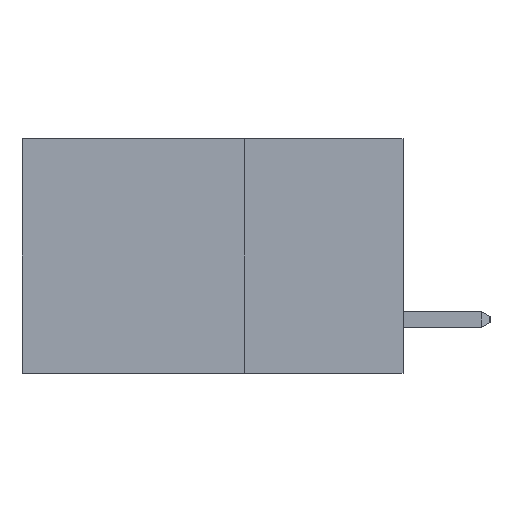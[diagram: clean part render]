
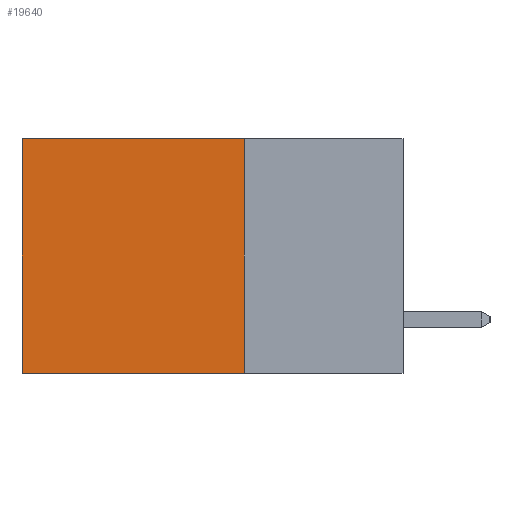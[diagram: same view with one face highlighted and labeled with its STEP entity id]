
A CAD part, left-side view. The second image highlights one B-rep face of the part: STEP entity #19640.
In plain terms, the highlighted planar face has unit normal (-1, 0, 0).
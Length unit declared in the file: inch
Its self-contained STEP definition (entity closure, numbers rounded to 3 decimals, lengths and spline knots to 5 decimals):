
#230 = EDGE_CURVE ( 'NONE', #2887, #5581, #7530, .T. ) ;
#419 = DIRECTION ( 'NONE',  ( 0., 1., 0. ) ) ;
#2053 = LINE ( 'NONE', #7343, #9746 ) ;
#2847 = LINE ( 'NONE', #5994, #10542 ) ;
#2887 = VERTEX_POINT ( 'NONE', #11896 ) ;
#3001 = ORIENTED_EDGE ( 'NONE', *, *, #4928, .F. ) ;
#3057 = VECTOR ( 'NONE', #419, 39.37008 ) ;
#4457 = CARTESIAN_POINT ( 'NONE',  ( 0.2875, 0.25, 0. ) ) ;
#4928 = EDGE_CURVE ( 'NONE', #5581, #10847, #2053, .T. ) ;
#5384 = ORIENTED_EDGE ( 'NONE', *, *, #10933, .T. ) ;
#5581 = VERTEX_POINT ( 'NONE', #11566 ) ;
#5994 = CARTESIAN_POINT ( 'NONE',  ( 0.2875, 0.6, 0. ) ) ;
#6035 = DIRECTION ( 'NONE',  ( 1., 0., 0. ) ) ;
#7012 = LINE ( 'NONE', #19492, #3057 ) ;
#7343 = CARTESIAN_POINT ( 'NONE',  ( 0.2875, 0.25, -0.37 ) ) ;
#7530 = LINE ( 'NONE', #17362, #8011 ) ;
#8011 = VECTOR ( 'NONE', #12726, 39.37008 ) ;
#8301 = CARTESIAN_POINT ( 'NONE',  ( 0.2875, 0.6, 0. ) ) ;
#8539 = FACE_OUTER_BOUND ( 'NONE', #18478, .T. ) ;
#9395 = DIRECTION ( 'NONE',  ( 0., 0., -1. ) ) ;
#9746 = VECTOR ( 'NONE', #11968, 39.37008 ) ;
#10028 = ORIENTED_EDGE ( 'NONE', *, *, #230, .F. ) ;
#10542 = VECTOR ( 'NONE', #9395, 39.37008 ) ;
#10847 = VERTEX_POINT ( 'NONE', #16704 ) ;
#10933 = EDGE_CURVE ( 'NONE', #18190, #10847, #2847, .T. ) ;
#11566 = CARTESIAN_POINT ( 'NONE',  ( 0.2875, 0.25, -0.37 ) ) ;
#11710 = AXIS2_PLACEMENT_3D ( 'NONE', #4457, #6035, #20407 ) ;
#11896 = CARTESIAN_POINT ( 'NONE',  ( 0.2875, 0.25, 0. ) ) ;
#11968 = DIRECTION ( 'NONE',  ( 0., 1., 0. ) ) ;
#12726 = DIRECTION ( 'NONE',  ( 0., 0., -1. ) ) ;
#15869 = EDGE_CURVE ( 'NONE', #2887, #18190, #7012, .T. ) ;
#16704 = CARTESIAN_POINT ( 'NONE',  ( 0.2875, 0.6, -0.37 ) ) ;
#16915 = ORIENTED_EDGE ( 'NONE', *, *, #15869, .T. ) ;
#17017 = PLANE ( 'NONE',  #11710 ) ;
#17362 = CARTESIAN_POINT ( 'NONE',  ( 0.2875, 0.25, 0. ) ) ;
#18190 = VERTEX_POINT ( 'NONE', #8301 ) ;
#18478 = EDGE_LOOP ( 'NONE', ( #5384, #3001, #10028, #16915 ) ) ;
#19492 = CARTESIAN_POINT ( 'NONE',  ( 0.2875, 0.25, 0. ) ) ;
#19640 = ADVANCED_FACE ( 'NONE', ( #8539 ), #17017, .F. ) ;
#20407 = DIRECTION ( 'NONE',  ( 0., 0., -1. ) ) ;
